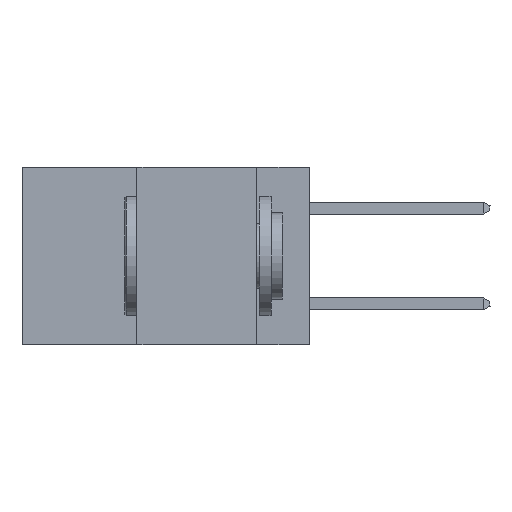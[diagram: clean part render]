
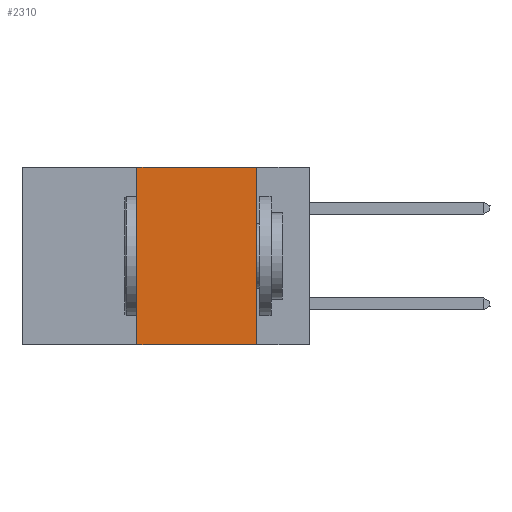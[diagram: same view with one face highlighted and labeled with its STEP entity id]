
A CAD part, left-side view. The second image highlights one B-rep face of the part: STEP entity #2310.
In plain terms, the highlighted planar face has unit normal (-1, 0, 0).
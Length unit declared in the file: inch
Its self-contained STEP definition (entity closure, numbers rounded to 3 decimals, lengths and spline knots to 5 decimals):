
#652 = DIRECTION ( 'NONE',  ( 0., -1., 0. ) ) ;
#988 = VECTOR ( 'NONE', #18016, 39.37008 ) ;
#1251 = EDGE_CURVE ( 'NONE', #4357, #20519, #6671, .T. ) ;
#1531 = VECTOR ( 'NONE', #7455, 39.37008 ) ;
#1640 = ORIENTED_EDGE ( 'NONE', *, *, #9721, .F. ) ;
#2171 = ORIENTED_EDGE ( 'NONE', *, *, #1251, .T. ) ;
#2310 = ADVANCED_FACE ( 'NONE', ( #9323 ), #21225, .F. ) ;
#4067 = ORIENTED_EDGE ( 'NONE', *, *, #24119, .F. ) ;
#4357 = VERTEX_POINT ( 'NONE', #21887 ) ;
#4560 = CARTESIAN_POINT ( 'NONE',  ( 0., 0.11, 0. ) ) ;
#6671 = LINE ( 'NONE', #9936, #1531 ) ;
#7455 = DIRECTION ( 'NONE',  ( 0., -1., 0. ) ) ;
#9323 = FACE_OUTER_BOUND ( 'NONE', #18195, .T. ) ;
#9502 = LINE ( 'NONE', #14067, #23446 ) ;
#9721 = EDGE_CURVE ( 'NONE', #14494, #10046, #9502, .T. ) ;
#9936 = CARTESIAN_POINT ( 'NONE',  ( 0., 0.6, -0.37 ) ) ;
#10046 = VERTEX_POINT ( 'NONE', #10319 ) ;
#10319 = CARTESIAN_POINT ( 'NONE',  ( 0., 0.11, 0. ) ) ;
#10670 = LINE ( 'NONE', #4560, #20202 ) ;
#11396 = EDGE_CURVE ( 'NONE', #4357, #14494, #16285, .T. ) ;
#14067 = CARTESIAN_POINT ( 'NONE',  ( 0., 0.6, 0. ) ) ;
#14221 = DIRECTION ( 'NONE',  ( 0., 0., -1. ) ) ;
#14494 = VERTEX_POINT ( 'NONE', #23455 ) ;
#16285 = LINE ( 'NONE', #23617, #988 ) ;
#17261 = CARTESIAN_POINT ( 'NONE',  ( 0., 0.11, -0.37 ) ) ;
#18016 = DIRECTION ( 'NONE',  ( 0., 0., 1. ) ) ;
#18195 = EDGE_LOOP ( 'NONE', ( #4067, #1640, #18442, #2171 ) ) ;
#18442 = ORIENTED_EDGE ( 'NONE', *, *, #11396, .F. ) ;
#19111 = AXIS2_PLACEMENT_3D ( 'NONE', #21282, #20824, #20635 ) ;
#20202 = VECTOR ( 'NONE', #14221, 39.37008 ) ;
#20519 = VERTEX_POINT ( 'NONE', #17261 ) ;
#20635 = DIRECTION ( 'NONE',  ( 0., 0., -1. ) ) ;
#20824 = DIRECTION ( 'NONE',  ( 1., 0., 0. ) ) ;
#21225 = PLANE ( 'NONE',  #19111 ) ;
#21282 = CARTESIAN_POINT ( 'NONE',  ( 0., 0.6, 0. ) ) ;
#21887 = CARTESIAN_POINT ( 'NONE',  ( 0., 0.36, -0.37 ) ) ;
#23446 = VECTOR ( 'NONE', #652, 39.37008 ) ;
#23455 = CARTESIAN_POINT ( 'NONE',  ( 0., 0.36, 0. ) ) ;
#23617 = CARTESIAN_POINT ( 'NONE',  ( 0., 0.36, 0. ) ) ;
#24119 = EDGE_CURVE ( 'NONE', #10046, #20519, #10670, .T. ) ;
